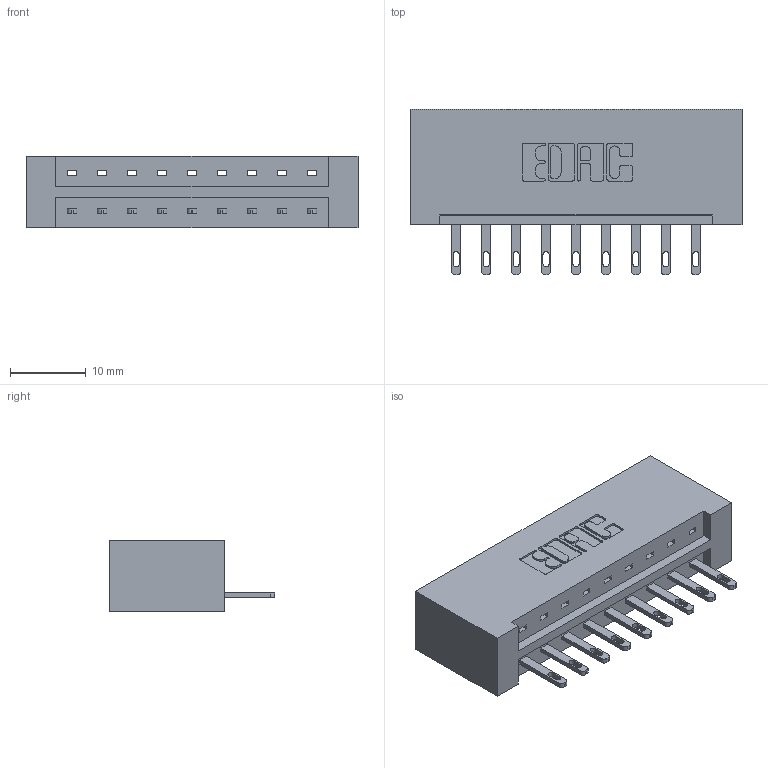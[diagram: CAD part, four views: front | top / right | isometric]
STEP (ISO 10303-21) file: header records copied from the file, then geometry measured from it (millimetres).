
FILE_DESCRIPTION (( 'STEP AP203' ), '1' );
FILE_NAME ('333-009-500-101.STEP', '2018-07-31T22:16:29', ( '' ), ( '' ), 'SwSTEP 2.0', 'SolidWorks 2016', '' );
FILE_SCHEMA (( 'CONFIG_CONTROL_DESIGN' ));
Length unit declared in the file: inch
Products named in the file (3): 333 Part_Lugless; 345-292-001_345-293-100; 333-009-500-101
Assembly tree (10 placements, depth 2):
  333-009-500-101
    333 Part_Lugless
    345-292-001_345-293-100  x9
Bounding box: 43.92 x 21.85 x 9.4 mm (x, y, z)
Volume: 4753.8 mm3; surface area: 4905.8 mm2
Topology: 10 solids, 10 shells, 592 faces, 1799 edges, 1198 vertices
Faces by surface type: plane 390, cylinder 202
Entity records: 9423 total; most frequent: CARTESIAN_POINT 1637, ORIENTED_EDGE 1582, DIRECTION 1441, EDGE_CURVE 791, VECTOR 667, LINE 667, VERTEX_POINT 526, AXIS2_PLACEMENT_3D 387
